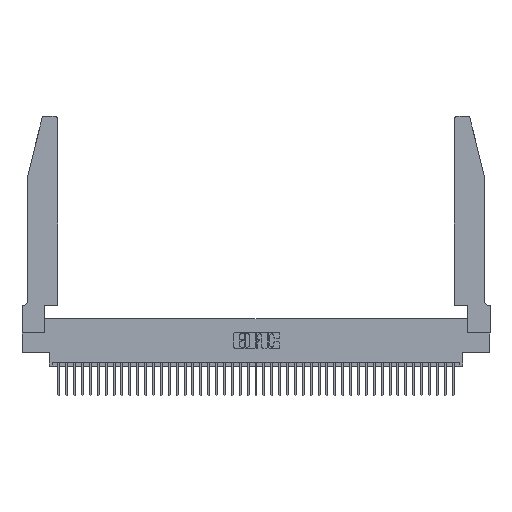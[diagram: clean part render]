
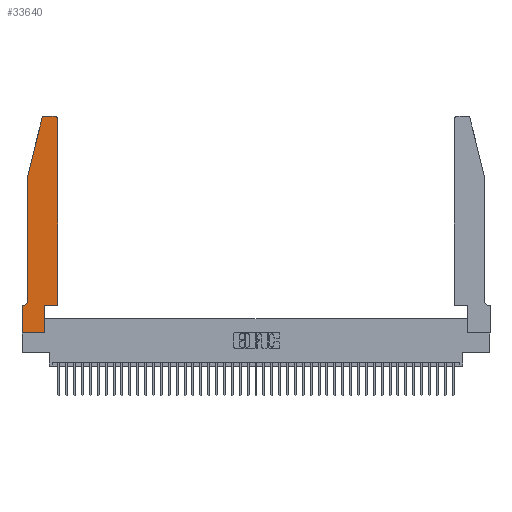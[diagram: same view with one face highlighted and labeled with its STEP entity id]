
A CAD part, top view. The second image highlights one B-rep face of the part: STEP entity #33640.
In plain terms, the highlighted planar face has unit normal (0, 0, 1).
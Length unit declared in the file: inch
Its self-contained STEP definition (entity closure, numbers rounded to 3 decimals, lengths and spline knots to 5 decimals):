
#67 = EDGE_LOOP ( 'NONE', ( #37431, #34052, #23426, #40861, #25686, #34630, #11175, #25473, #32847, #3356, #14546, #29223 ) ) ;
#150 = EDGE_CURVE ( 'NONE', #36809, #26513, #20513, .T. ) ;
#265 = AXIS2_PLACEMENT_3D ( 'NONE', #7952, #24534, #17558 ) ;
#349 = EDGE_CURVE ( 'NONE', #38746, #18234, #10428, .T. ) ;
#882 = PLANE ( 'NONE',  #265 ) ;
#922 = DIRECTION ( 'NONE',  ( 0., 0., 1. ) ) ;
#1483 = VECTOR ( 'NONE', #16048, 39.37008 ) ;
#1597 = CARTESIAN_POINT ( 'NONE',  ( 0.0055, 0.42, 0.37 ) ) ;
#2054 = DIRECTION ( 'NONE',  ( 0., 0., 1. ) ) ;
#2741 = CARTESIAN_POINT ( 'NONE',  ( 0.0755, 2., 0.37 ) ) ;
#2897 = CARTESIAN_POINT ( 'NONE',  ( 0.4505, 0.35, 0.37 ) ) ;
#3356 = ORIENTED_EDGE ( 'NONE', *, *, #20034, .T. ) ;
#3702 = VERTEX_POINT ( 'NONE', #38862 ) ;
#3727 = FACE_OUTER_BOUND ( 'NONE', #67, .T. ) ;
#3841 = EDGE_CURVE ( 'NONE', #23659, #18749, #9295, .T. ) ;
#5228 = VECTOR ( 'NONE', #11320, 39.37008 ) ;
#6243 = CARTESIAN_POINT ( 'NONE',  ( 0., 0., 0.37 ) ) ;
#6532 = CARTESIAN_POINT ( 'NONE',  ( 0.4505, 2.72, 0.37 ) ) ;
#7354 = LINE ( 'NONE', #34960, #5228 ) ;
#7688 = DIRECTION ( 'NONE',  ( 1., 0., 0. ) ) ;
#7952 = CARTESIAN_POINT ( 'NONE',  ( 0., 0.35, 0.37 ) ) ;
#8896 = LINE ( 'NONE', #36415, #9973 ) ;
#9295 = LINE ( 'NONE', #16185, #10357 ) ;
#9973 = VECTOR ( 'NONE', #22954, 39.37008 ) ;
#10148 = EDGE_CURVE ( 'NONE', #30690, #36809, #26575, .T. ) ;
#10357 = VECTOR ( 'NONE', #39852, 39.37008 ) ;
#10428 = LINE ( 'NONE', #2741, #1483 ) ;
#10825 = LINE ( 'NONE', #2897, #12973 ) ;
#11175 = ORIENTED_EDGE ( 'NONE', *, *, #23780, .T. ) ;
#11320 = DIRECTION ( 'NONE',  ( 0., -1., 0. ) ) ;
#12357 = AXIS2_PLACEMENT_3D ( 'NONE', #1597, #18139, #18577 ) ;
#12973 = VECTOR ( 'NONE', #16345, 39.37008 ) ;
#14125 = AXIS2_PLACEMENT_3D ( 'NONE', #16218, #2054, #32919 ) ;
#14546 = ORIENTED_EDGE ( 'NONE', *, *, #17892, .T. ) ;
#14743 = DIRECTION ( 'NONE',  ( -1., 0., 0. ) ) ;
#15227 = CARTESIAN_POINT ( 'NONE',  ( 0.2865, 0.35, 0.37 ) ) ;
#15772 = DIRECTION ( 'NONE',  ( 0., -1., 0. ) ) ;
#16048 = DIRECTION ( 'NONE',  ( -0.239, -0.971, 0. ) ) ;
#16185 = CARTESIAN_POINT ( 'NONE',  ( 0.2605, 2.75, 0.37 ) ) ;
#16218 = CARTESIAN_POINT ( 'NONE',  ( 0.284, 2.72, 0.37 ) ) ;
#16345 = DIRECTION ( 'NONE',  ( 1., 0., 0. ) ) ;
#16898 = VERTEX_POINT ( 'NONE', #6243 ) ;
#17558 = DIRECTION ( 'NONE',  ( 1., 0., 0. ) ) ;
#17759 = VECTOR ( 'NONE', #22236, 39.37008 ) ;
#17892 = EDGE_CURVE ( 'NONE', #42024, #18637, #8896, .T. ) ;
#18139 = DIRECTION ( 'NONE',  ( 0., 0., -1. ) ) ;
#18234 = VERTEX_POINT ( 'NONE', #29633 ) ;
#18577 = DIRECTION ( 'NONE',  ( -1., 0., 0. ) ) ;
#18637 = VERTEX_POINT ( 'NONE', #6532 ) ;
#18749 = VERTEX_POINT ( 'NONE', #42263 ) ;
#19086 = VECTOR ( 'NONE', #41564, 39.37008 ) ;
#19178 = CARTESIAN_POINT ( 'NONE',  ( 0.4505, 0.35, 0.37 ) ) ;
#20034 = EDGE_CURVE ( 'NONE', #3702, #42024, #10825, .T. ) ;
#20241 = EDGE_CURVE ( 'NONE', #16898, #27308, #43633, .T. ) ;
#20513 = LINE ( 'NONE', #30567, #29495 ) ;
#21163 = CIRCLE ( 'NONE', #14125, 0.03 ) ;
#22103 = CARTESIAN_POINT ( 'NONE',  ( 0., 0., 0.37 ) ) ;
#22236 = DIRECTION ( 'NONE',  ( 1., 0., 0. ) ) ;
#22954 = DIRECTION ( 'NONE',  ( 0., 1., 0. ) ) ;
#23076 = EDGE_CURVE ( 'NONE', #27308, #3702, #28063, .T. ) ;
#23426 = ORIENTED_EDGE ( 'NONE', *, *, #349, .T. ) ;
#23659 = VERTEX_POINT ( 'NONE', #40473 ) ;
#23780 = EDGE_CURVE ( 'NONE', #26513, #16898, #7354, .T. ) ;
#24534 = DIRECTION ( 'NONE',  ( 0., 0., 1. ) ) ;
#25241 = CARTESIAN_POINT ( 'NONE',  ( 0.25487, 2.72718, 0.37 ) ) ;
#25327 = CIRCLE ( 'NONE', #25806, 0.03 ) ;
#25473 = ORIENTED_EDGE ( 'NONE', *, *, #20241, .T. ) ;
#25686 = ORIENTED_EDGE ( 'NONE', *, *, #10148, .T. ) ;
#25806 = AXIS2_PLACEMENT_3D ( 'NONE', #34458, #922, #7688 ) ;
#26513 = VERTEX_POINT ( 'NONE', #38037 ) ;
#26575 = CIRCLE ( 'NONE', #12357, 0.07 ) ;
#26836 = VECTOR ( 'NONE', #15772, 39.37008 ) ;
#27276 = EDGE_CURVE ( 'NONE', #18749, #38746, #21163, .T. ) ;
#27308 = VERTEX_POINT ( 'NONE', #35898 ) ;
#28063 = LINE ( 'NONE', #15227, #19086 ) ;
#28349 = EDGE_CURVE ( 'NONE', #18637, #23659, #25327, .T. ) ;
#28467 = CARTESIAN_POINT ( 'NONE',  ( 0.0755, 2., 0.37 ) ) ;
#29223 = ORIENTED_EDGE ( 'NONE', *, *, #28349, .T. ) ;
#29252 = EDGE_CURVE ( 'NONE', #18234, #30690, #32680, .T. ) ;
#29495 = VECTOR ( 'NONE', #14743, 39.37008 ) ;
#29633 = CARTESIAN_POINT ( 'NONE',  ( 0.0755, 2., 0.37 ) ) ;
#30567 = CARTESIAN_POINT ( 'NONE',  ( 0.0755, 0.35, 0.37 ) ) ;
#30690 = VERTEX_POINT ( 'NONE', #38380 ) ;
#31921 = CARTESIAN_POINT ( 'NONE',  ( 0.0055, 0.35, 0.37 ) ) ;
#32680 = LINE ( 'NONE', #28467, #26836 ) ;
#32847 = ORIENTED_EDGE ( 'NONE', *, *, #23076, .T. ) ;
#32919 = DIRECTION ( 'NONE',  ( 1., 0., 0. ) ) ;
#33640 = ADVANCED_FACE ( 'NONE', ( #3727 ), #882, .T. ) ;
#34052 = ORIENTED_EDGE ( 'NONE', *, *, #27276, .T. ) ;
#34458 = CARTESIAN_POINT ( 'NONE',  ( 0.4205, 2.72, 0.37 ) ) ;
#34630 = ORIENTED_EDGE ( 'NONE', *, *, #150, .T. ) ;
#34960 = CARTESIAN_POINT ( 'NONE',  ( 0., 0., 0.37 ) ) ;
#35898 = CARTESIAN_POINT ( 'NONE',  ( 0.2865, 0., 0.37 ) ) ;
#36415 = CARTESIAN_POINT ( 'NONE',  ( 0.4505, 0.35, 0.37 ) ) ;
#36809 = VERTEX_POINT ( 'NONE', #31921 ) ;
#37431 = ORIENTED_EDGE ( 'NONE', *, *, #3841, .T. ) ;
#38037 = CARTESIAN_POINT ( 'NONE',  ( 0., 0.35, 0.37 ) ) ;
#38380 = CARTESIAN_POINT ( 'NONE',  ( 0.0755, 0.42, 0.37 ) ) ;
#38746 = VERTEX_POINT ( 'NONE', #25241 ) ;
#38862 = CARTESIAN_POINT ( 'NONE',  ( 0.2865, 0.35, 0.37 ) ) ;
#39852 = DIRECTION ( 'NONE',  ( -1., 0., 0. ) ) ;
#40473 = CARTESIAN_POINT ( 'NONE',  ( 0.4205, 2.75, 0.37 ) ) ;
#40861 = ORIENTED_EDGE ( 'NONE', *, *, #29252, .T. ) ;
#41564 = DIRECTION ( 'NONE',  ( 0., 1., 0. ) ) ;
#42024 = VERTEX_POINT ( 'NONE', #19178 ) ;
#42263 = CARTESIAN_POINT ( 'NONE',  ( 0.284, 2.75, 0.37 ) ) ;
#43633 = LINE ( 'NONE', #22103, #17759 ) ;
